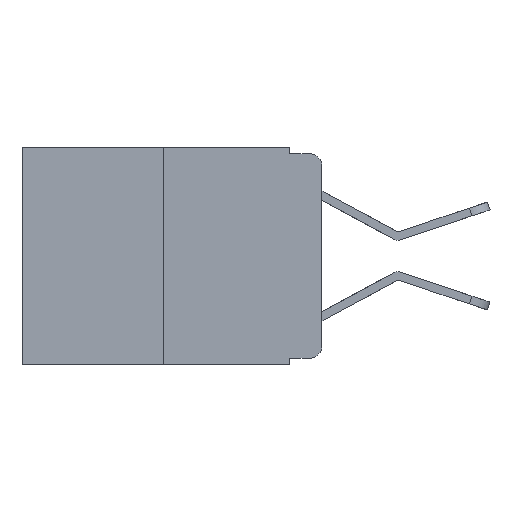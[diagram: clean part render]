
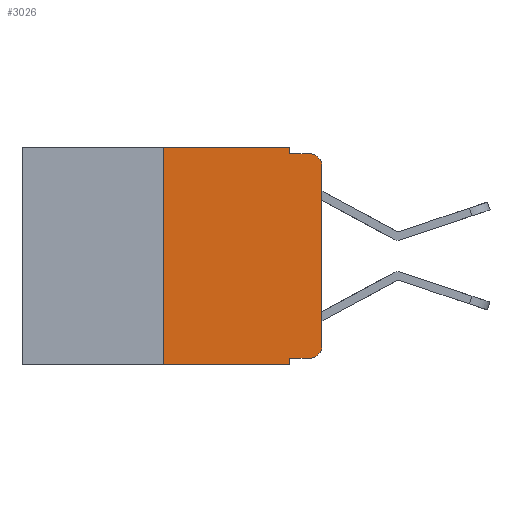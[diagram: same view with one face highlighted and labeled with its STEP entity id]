
A CAD part, left-side view. The second image highlights one B-rep face of the part: STEP entity #3026.
In plain terms, the highlighted planar face has unit normal (-1, 0, 0).
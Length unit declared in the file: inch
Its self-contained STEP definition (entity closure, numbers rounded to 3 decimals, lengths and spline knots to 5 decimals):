
#199 = CARTESIAN_POINT ( 'NONE',  ( 0., 0.051, 0. ) ) ;
#212 = CARTESIAN_POINT ( 'NONE',  ( 0., 0.25, 0. ) ) ;
#600 = VERTEX_POINT ( 'NONE', #2226 ) ;
#618 = DIRECTION ( 'NONE',  ( 0., -1., 0. ) ) ;
#681 = CARTESIAN_POINT ( 'NONE',  ( 0., 0.051, 0. ) ) ;
#907 = EDGE_CURVE ( 'NONE', #8977, #8728, #4116, .T. ) ;
#922 = VERTEX_POINT ( 'NONE', #12590 ) ;
#1198 = LINE ( 'NONE', #10219, #2925 ) ;
#1453 = ORIENTED_EDGE ( 'NONE', *, *, #10814, .F. ) ;
#1494 = DIRECTION ( 'NONE',  ( 0., -1., 0. ) ) ;
#1550 = CARTESIAN_POINT ( 'NONE',  ( 0., 0.25, 0. ) ) ;
#1590 = CARTESIAN_POINT ( 'NONE',  ( 0., 0.051, -0.01 ) ) ;
#1602 = ORIENTED_EDGE ( 'NONE', *, *, #907, .F. ) ;
#1639 = EDGE_CURVE ( 'NONE', #11399, #922, #9158, .T. ) ;
#1919 = ORIENTED_EDGE ( 'NONE', *, *, #7276, .F. ) ;
#2009 = CIRCLE ( 'NONE', #4427, 0.02 ) ;
#2098 = ORIENTED_EDGE ( 'NONE', *, *, #1639, .T. ) ;
#2226 = CARTESIAN_POINT ( 'NONE',  ( 0., 0.25, -0.343 ) ) ;
#2329 = VECTOR ( 'NONE', #618, 39.37008 ) ;
#2433 = DIRECTION ( 'NONE',  ( -1., 0., 0. ) ) ;
#2870 = ORIENTED_EDGE ( 'NONE', *, *, #7519, .F. ) ;
#2925 = VECTOR ( 'NONE', #5382, 39.37008 ) ;
#3026 = ADVANCED_FACE ( 'NONE', ( #9122 ), #3432, .F. ) ;
#3432 = PLANE ( 'NONE',  #10211 ) ;
#3514 = DIRECTION ( 'NONE',  ( 0., 0., 1. ) ) ;
#3640 = EDGE_CURVE ( 'NONE', #11931, #10788, #9841, .T. ) ;
#4010 = EDGE_CURVE ( 'NONE', #10056, #8728, #10400, .T. ) ;
#4116 = LINE ( 'NONE', #1590, #11494 ) ;
#4416 = DIRECTION ( 'NONE',  ( 0., 0., -1. ) ) ;
#4427 = AXIS2_PLACEMENT_3D ( 'NONE', #8328, #2433, #9317 ) ;
#4597 = CARTESIAN_POINT ( 'NONE',  ( 0., 0.051, 0. ) ) ;
#4810 = EDGE_CURVE ( 'NONE', #922, #6546, #2009, .T. ) ;
#5161 = CARTESIAN_POINT ( 'NONE',  ( 0., 0.02, -0.03 ) ) ;
#5170 = ORIENTED_EDGE ( 'NONE', *, *, #3640, .F. ) ;
#5305 = CARTESIAN_POINT ( 'NONE',  ( 0., 0.051, -0.343 ) ) ;
#5382 = DIRECTION ( 'NONE',  ( 0., 0., 1. ) ) ;
#5445 = DIRECTION ( 'NONE',  ( 0., -1., 0. ) ) ;
#6157 = DIRECTION ( 'NONE',  ( 0., 0., -1. ) ) ;
#6192 = DIRECTION ( 'NONE',  ( 0., 0., -1. ) ) ;
#6546 = VERTEX_POINT ( 'NONE', #7042 ) ;
#6657 = DIRECTION ( 'NONE',  ( 0., 0., -1. ) ) ;
#6751 = VECTOR ( 'NONE', #6657, 39.37008 ) ;
#7042 = CARTESIAN_POINT ( 'NONE',  ( 0., 0., -0.313 ) ) ;
#7276 = EDGE_CURVE ( 'NONE', #10788, #8977, #10610, .T. ) ;
#7303 = VECTOR ( 'NONE', #3514, 39.37008 ) ;
#7343 = CARTESIAN_POINT ( 'NONE',  ( 0., 0.473, 0. ) ) ;
#7395 = CARTESIAN_POINT ( 'NONE',  ( 0., 0.473, -0.343 ) ) ;
#7448 = EDGE_CURVE ( 'NONE', #600, #8059, #10753, .T. ) ;
#7456 = VECTOR ( 'NONE', #6192, 39.37008 ) ;
#7458 = EDGE_LOOP ( 'NONE', ( #10779, #11064, #1602, #1919, #5170, #2870, #8725, #1453, #2098, #12378 ) ) ;
#7519 = EDGE_CURVE ( 'NONE', #600, #11931, #7608, .T. ) ;
#7608 = LINE ( 'NONE', #1550, #7303 ) ;
#7767 = CARTESIAN_POINT ( 'NONE',  ( 0., 0.051, -0.333 ) ) ;
#8059 = VERTEX_POINT ( 'NONE', #5305 ) ;
#8255 = CARTESIAN_POINT ( 'NONE',  ( 0., 0.02, -0.01 ) ) ;
#8328 = CARTESIAN_POINT ( 'NONE',  ( 0., 0.02, -0.313 ) ) ;
#8725 = ORIENTED_EDGE ( 'NONE', *, *, #7448, .T. ) ;
#8728 = VERTEX_POINT ( 'NONE', #8255 ) ;
#8818 = DIRECTION ( 'NONE',  ( 0., -1., 0. ) ) ;
#8834 = CARTESIAN_POINT ( 'NONE',  ( 0., 0.051, -0.333 ) ) ;
#8977 = VERTEX_POINT ( 'NONE', #9522 ) ;
#9122 = FACE_OUTER_BOUND ( 'NONE', #7458, .T. ) ;
#9158 = LINE ( 'NONE', #8834, #11049 ) ;
#9317 = DIRECTION ( 'NONE',  ( 0., 0., -1. ) ) ;
#9522 = CARTESIAN_POINT ( 'NONE',  ( 0., 0.051, -0.01 ) ) ;
#9841 = LINE ( 'NONE', #12263, #2329 ) ;
#10027 = EDGE_CURVE ( 'NONE', #6546, #10056, #1198, .T. ) ;
#10056 = VERTEX_POINT ( 'NONE', #12052 ) ;
#10211 = AXIS2_PLACEMENT_3D ( 'NONE', #7343, #10241, #4416 ) ;
#10218 = LINE ( 'NONE', #681, #6751 ) ;
#10219 = CARTESIAN_POINT ( 'NONE',  ( 0., 0., 0. ) ) ;
#10241 = DIRECTION ( 'NONE',  ( 1., 0., 0. ) ) ;
#10400 = CIRCLE ( 'NONE', #12632, 0.02 ) ;
#10443 = VECTOR ( 'NONE', #5445, 39.37008 ) ;
#10610 = LINE ( 'NONE', #199, #7456 ) ;
#10753 = LINE ( 'NONE', #7395, #10443 ) ;
#10779 = ORIENTED_EDGE ( 'NONE', *, *, #10027, .T. ) ;
#10788 = VERTEX_POINT ( 'NONE', #4597 ) ;
#10814 = EDGE_CURVE ( 'NONE', #11399, #8059, #10218, .T. ) ;
#11049 = VECTOR ( 'NONE', #8818, 39.37008 ) ;
#11064 = ORIENTED_EDGE ( 'NONE', *, *, #4010, .T. ) ;
#11399 = VERTEX_POINT ( 'NONE', #7767 ) ;
#11494 = VECTOR ( 'NONE', #1494, 39.37008 ) ;
#11894 = DIRECTION ( 'NONE',  ( -1., 0., 0. ) ) ;
#11931 = VERTEX_POINT ( 'NONE', #212 ) ;
#12052 = CARTESIAN_POINT ( 'NONE',  ( 0., 0., -0.03 ) ) ;
#12263 = CARTESIAN_POINT ( 'NONE',  ( 0., 0.473, 0. ) ) ;
#12378 = ORIENTED_EDGE ( 'NONE', *, *, #4810, .T. ) ;
#12590 = CARTESIAN_POINT ( 'NONE',  ( 0., 0.02, -0.333 ) ) ;
#12632 = AXIS2_PLACEMENT_3D ( 'NONE', #5161, #11894, #6157 ) ;
